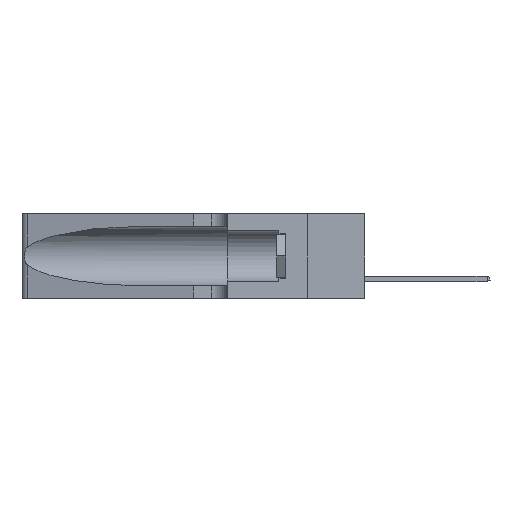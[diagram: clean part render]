
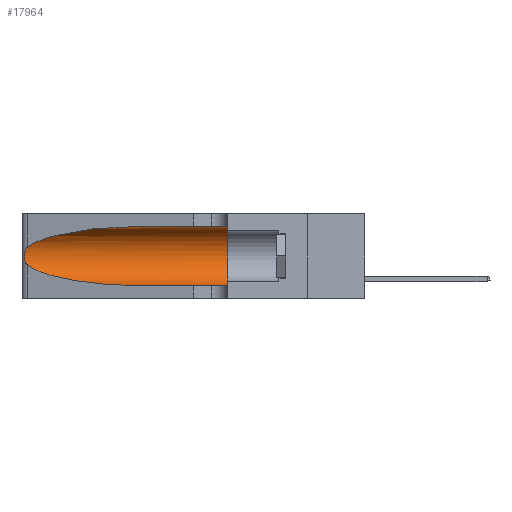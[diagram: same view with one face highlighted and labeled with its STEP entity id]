
A CAD part, left-side view. The second image highlights one B-rep face of the part: STEP entity #17964.
In plain terms, the highlighted cylindrical face has radius 3.308 mm (diameter 6.617 mm), a partial arc.
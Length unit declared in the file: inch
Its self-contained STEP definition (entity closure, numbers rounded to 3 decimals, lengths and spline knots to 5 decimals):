
#130 = DIRECTION ( 'NONE',  ( 0., -1., 0. ) ) ;
#359 = VERTEX_POINT ( 'NONE', #11805 ) ;
#1467 = LINE ( 'NONE', #32267, #33236 ) ;
#1598 = CARTESIAN_POINT ( 'NONE',  ( 0.25555, 1.22993, 0.14849 ) ) ;
#2119 = CARTESIAN_POINT ( 'NONE',  ( 0.25639, 1.23184, 0.21858 ) ) ;
#2717 = CARTESIAN_POINT ( 'NONE',  ( 0.1305, 0.72297, 0.05475 ) ) ;
#4703 = CARTESIAN_POINT ( 'NONE',  ( 0.25639, 1.23186, 0.15144 ) ) ;
#4950 = CARTESIAN_POINT ( 'NONE',  ( 0.25487, 1.22718, 0.14631 ) ) ;
#6999 = DIRECTION ( 'NONE',  ( 0., 0., 1. ) ) ;
#7278 = B_SPLINE_CURVE_WITH_KNOTS ( 'NONE', 3,
 ( #36842, #33898, #2119, #34427, #37249, #22213, #37107, #25699, #25451, #10730, #27975, #4703, #1598, #4950 ),
 .UNSPECIFIED., .F., .F.,
 ( 4, 2, 2, 2, 2, 2, 4 ),
 ( 0., 0.00027, 0.00053, 0.00107, 0.0016, 0.00187, 0.00214 ),
 .UNSPECIFIED. ) ;
#7549 = VERTEX_POINT ( 'NONE', #34726 ) ;
#8245 =( BOUNDED_CURVE ( )  B_SPLINE_CURVE ( 3, ( #26916, #11840, #8917, #17913 ),
 .UNSPECIFIED., .F., .F. ) 
 B_SPLINE_CURVE_WITH_KNOTS ( ( 4, 4 ),
 ( 1.5708, 2.84003 ),
 .UNSPECIFIED. ) 
 CURVE ( )  GEOMETRIC_REPRESENTATION_ITEM ( )  RATIONAL_B_SPLINE_CURVE ( ( 1., 0.87, 0.87, 1. ) ) 
 REPRESENTATION_ITEM ( '' )  );
#8542 = FACE_OUTER_BOUND ( 'NONE', #14996, .T. ) ;
#8917 = CARTESIAN_POINT ( 'NONE',  ( 0.2373, 1.15595, 0.28018 ) ) ;
#10052 = DIRECTION ( 'NONE',  ( 0., -1., 0. ) ) ;
#10309 = DIRECTION ( 'NONE',  ( 0., 1., 0. ) ) ;
#10730 = CARTESIAN_POINT ( 'NONE',  ( 0.25856, 1.23593, 0.16098 ) ) ;
#11290 = CARTESIAN_POINT ( 'NONE',  ( 0.18966, 0.96281, 0.05475 ) ) ;
#11805 = CARTESIAN_POINT ( 'NONE',  ( 0.1305, 0.72297, 0.05475 ) ) ;
#11840 = CARTESIAN_POINT ( 'NONE',  ( 0.18966, 0.96281, 0.31525 ) ) ;
#12573 = VERTEX_POINT ( 'NONE', #21593 ) ;
#13423 = DIRECTION ( 'NONE',  ( 0., 0., -1. ) ) ;
#14827 = AXIS2_PLACEMENT_3D ( 'NONE', #22187, #10309, #6999 ) ;
#14996 = EDGE_LOOP ( 'NONE', ( #36210, #30664, #16013, #18098, #36400, #37384 ) ) ;
#15164 = CARTESIAN_POINT ( 'NONE',  ( 0.1305, 0.72297, 0.31525 ) ) ;
#16013 = ORIENTED_EDGE ( 'NONE', *, *, #19150, .T. ) ;
#16182 = EDGE_CURVE ( 'NONE', #12573, #7549, #22185, .T. ) ;
#16998 = CARTESIAN_POINT ( 'NONE',  ( 0.25487, 1.22718, 0.14631 ) ) ;
#17913 = CARTESIAN_POINT ( 'NONE',  ( 0.25487, 1.22718, 0.22369 ) ) ;
#17964 = ADVANCED_FACE ( 'NONE', ( #8542 ), #32859, .F. ) ;
#18098 = ORIENTED_EDGE ( 'NONE', *, *, #36620, .T. ) ;
#18671 = EDGE_CURVE ( 'NONE', #35416, #32238, #7278, .T. ) ;
#19064 = CARTESIAN_POINT ( 'NONE',  ( 0.1305, 1.61858, 0.185 ) ) ;
#19150 = EDGE_CURVE ( 'NONE', #32238, #359, #29886, .T. ) ;
#21186 = CARTESIAN_POINT ( 'NONE',  ( 0.25487, 1.22718, 0.22369 ) ) ;
#21593 = CARTESIAN_POINT ( 'NONE',  ( 0.1305, 0.35, 0.31525 ) ) ;
#22185 = CIRCLE ( 'NONE', #14827, 0.13025 ) ;
#22187 = CARTESIAN_POINT ( 'NONE',  ( 0.1305, 0.35, 0.185 ) ) ;
#22213 = CARTESIAN_POINT ( 'NONE',  ( 0.26018, 1.23835, 0.19895 ) ) ;
#22220 = VECTOR ( 'NONE', #10052, 39.37008 ) ;
#23049 = CARTESIAN_POINT ( 'NONE',  ( 0.2373, 1.15595, 0.08982 ) ) ;
#25196 = DIRECTION ( 'NONE',  ( 0., -1., 0. ) ) ;
#25451 = CARTESIAN_POINT ( 'NONE',  ( 0.26017, 1.23833, 0.17102 ) ) ;
#25699 = CARTESIAN_POINT ( 'NONE',  ( 0.26075, 1.23896, 0.178 ) ) ;
#26916 = CARTESIAN_POINT ( 'NONE',  ( 0.1305, 0.72297, 0.31525 ) ) ;
#27975 = CARTESIAN_POINT ( 'NONE',  ( 0.25789, 1.23486, 0.15765 ) ) ;
#28830 = VERTEX_POINT ( 'NONE', #15164 ) ;
#29886 =( BOUNDED_CURVE ( )  B_SPLINE_CURVE ( 3, ( #16998, #23049, #11290, #2717 ),
 .UNSPECIFIED., .F., .F. ) 
 B_SPLINE_CURVE_WITH_KNOTS ( ( 4, 4 ),
 ( 3.44316, 4.71239 ),
 .UNSPECIFIED. ) 
 CURVE ( )  GEOMETRIC_REPRESENTATION_ITEM ( )  RATIONAL_B_SPLINE_CURVE ( ( 1., 0.87, 0.87, 1. ) ) 
 REPRESENTATION_ITEM ( '' )  );
#30664 = ORIENTED_EDGE ( 'NONE', *, *, #18671, .T. ) ;
#32238 = VERTEX_POINT ( 'NONE', #32286 ) ;
#32267 = CARTESIAN_POINT ( 'NONE',  ( 0.1305, 1.61858, 0.05475 ) ) ;
#32286 = CARTESIAN_POINT ( 'NONE',  ( 0.25487, 1.22718, 0.14631 ) ) ;
#32859 = CYLINDRICAL_SURFACE ( 'NONE', #37567, 0.13025 ) ;
#33236 = VECTOR ( 'NONE', #130, 39.37008 ) ;
#33898 = CARTESIAN_POINT ( 'NONE',  ( 0.25555, 1.22994, 0.2215 ) ) ;
#34146 = EDGE_CURVE ( 'NONE', #28830, #35416, #8245, .T. ) ;
#34427 = CARTESIAN_POINT ( 'NONE',  ( 0.25787, 1.23484, 0.2124 ) ) ;
#34726 = CARTESIAN_POINT ( 'NONE',  ( 0.1305, 0.35, 0.05475 ) ) ;
#35416 = VERTEX_POINT ( 'NONE', #21186 ) ;
#36210 = ORIENTED_EDGE ( 'NONE', *, *, #34146, .T. ) ;
#36400 = ORIENTED_EDGE ( 'NONE', *, *, #16182, .F. ) ;
#36620 = EDGE_CURVE ( 'NONE', #359, #7549, #1467, .T. ) ;
#36680 = CARTESIAN_POINT ( 'NONE',  ( 0.1305, 1.61858, 0.31525 ) ) ;
#36842 = CARTESIAN_POINT ( 'NONE',  ( 0.25487, 1.22718, 0.22369 ) ) ;
#37107 = CARTESIAN_POINT ( 'NONE',  ( 0.26075, 1.23896, 0.19203 ) ) ;
#37249 = CARTESIAN_POINT ( 'NONE',  ( 0.25854, 1.2359, 0.20912 ) ) ;
#37251 = EDGE_CURVE ( 'NONE', #28830, #12573, #37871, .T. ) ;
#37384 = ORIENTED_EDGE ( 'NONE', *, *, #37251, .F. ) ;
#37567 = AXIS2_PLACEMENT_3D ( 'NONE', #19064, #25196, #13423 ) ;
#37871 = LINE ( 'NONE', #36680, #22220 ) ;
